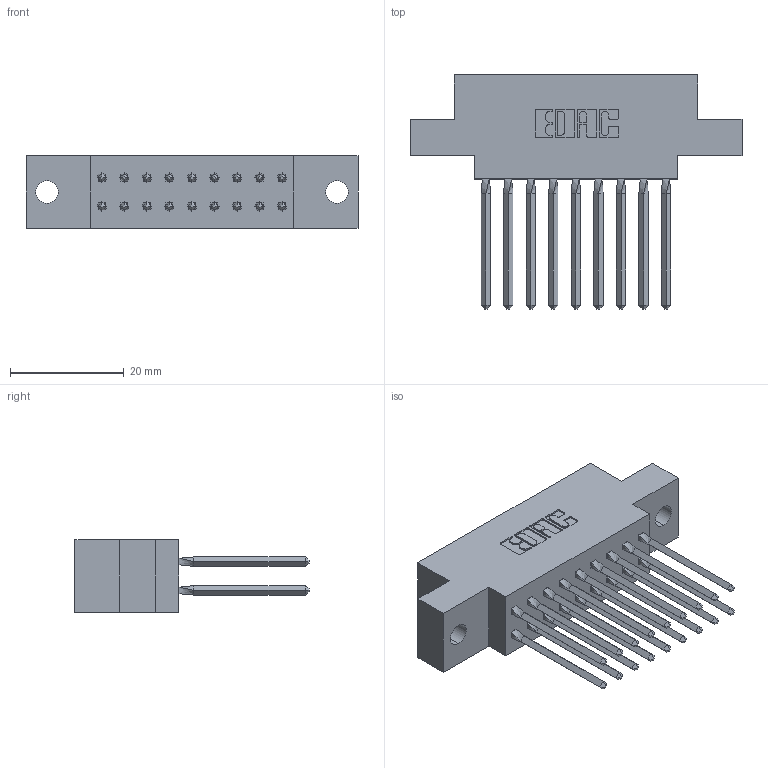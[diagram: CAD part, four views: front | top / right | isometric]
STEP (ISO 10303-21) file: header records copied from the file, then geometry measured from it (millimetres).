
FILE_DESCRIPTION (( 'STEP AP203' ), '1' );
FILE_NAME ('317-018-543-804.STEP', '2020-02-27T16:12:16', ( '' ), ( '' ), 'SwSTEP 2.0', 'SolidWorks 2016', '' );
FILE_SCHEMA (( 'CONFIG_CONTROL_DESIGN' ));
Length unit declared in the file: inch
Products named in the file (3): 317 Part_.156 Dia - TH; 317-290-001_543; 317-018-543-804
Assembly tree (19 placements, depth 2):
  317-018-543-804
    317 Part_.156 Dia - TH
    317-290-001_543  x18
Bounding box: 58.37 x 41.15 x 12.7 mm (x, y, z)
Volume: 8682.1 mm3; surface area: 11702.7 mm2
Topology: 19 solids, 19 shells, 1704 faces, 4721 edges, 3044 vertices
Faces by surface type: plane 1372, cylinder 260, bspline 72
Entity records: 17616 total; most frequent: CARTESIAN_POINT 3483, ORIENTED_EDGE 2982, DIRECTION 2493, EDGE_CURVE 1491, LINE 1235, VECTOR 1235, VERTEX_POINT 987, AXIS2_PLACEMENT_3D 629
